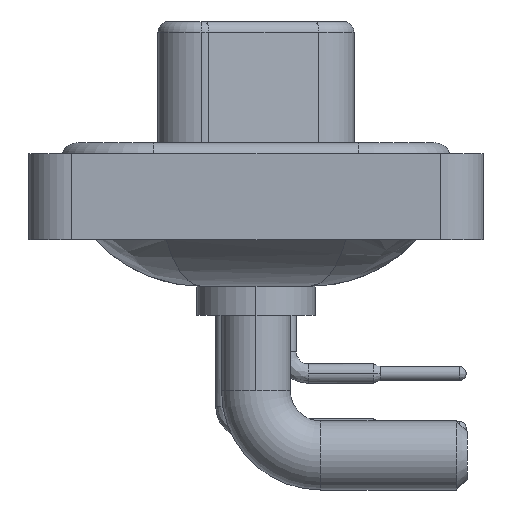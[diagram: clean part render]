
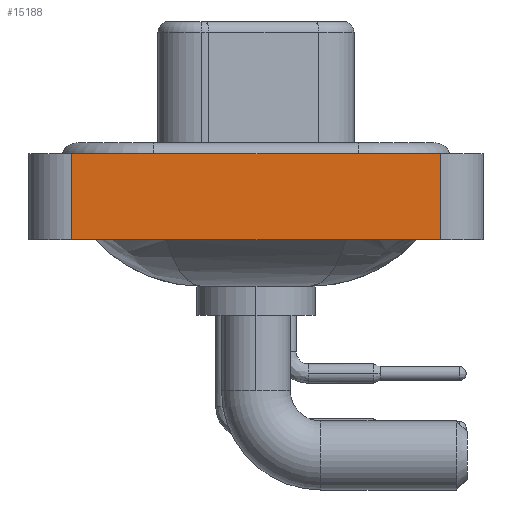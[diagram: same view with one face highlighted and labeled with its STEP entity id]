
A CAD part, left-side view. The second image highlights one B-rep face of the part: STEP entity #15188.
In plain terms, the highlighted planar face has unit normal (-1, 0, 0).
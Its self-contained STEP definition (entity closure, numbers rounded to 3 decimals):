
#983 = DIRECTION ( 'NONE',  ( -1., 0., 0. ) ) ;
#1183 = CARTESIAN_POINT ( 'NONE',  ( -7.35, -8.55, 0.4 ) ) ;
#1328 = EDGE_CURVE ( 'NONE', #18707, #13131, #21743, .T. ) ;
#1585 = EDGE_CURVE ( 'NONE', #18707, #22720, #2840, .T. ) ;
#2404 = EDGE_LOOP ( 'NONE', ( #7082, #12515, #13923, #10866 ) ) ;
#2840 = LINE ( 'NONE', #12979, #15301 ) ;
#2949 = FACE_OUTER_BOUND ( 'NONE', #2404, .T. ) ;
#3801 = VECTOR ( 'NONE', #6487, 1000. ) ;
#5107 = DIRECTION ( 'NONE',  ( 0., 0., 1. ) ) ;
#6487 = DIRECTION ( 'NONE',  ( 0., -1., 0. ) ) ;
#6903 = CARTESIAN_POINT ( 'NONE',  ( -7.35, -8.55, -3.6 ) ) ;
#7082 = ORIENTED_EDGE ( 'NONE', *, *, #14349, .T. ) ;
#7243 = CARTESIAN_POINT ( 'NONE',  ( -7.35, 8.55, -3.6 ) ) ;
#9019 = DIRECTION ( 'NONE',  ( 0., 0., 1. ) ) ;
#9281 = PLANE ( 'NONE',  #21381 ) ;
#10866 = ORIENTED_EDGE ( 'NONE', *, *, #1585, .T. ) ;
#11995 = EDGE_CURVE ( 'NONE', #13131, #23366, #19168, .T. ) ;
#12515 = ORIENTED_EDGE ( 'NONE', *, *, #11995, .F. ) ;
#12979 = CARTESIAN_POINT ( 'NONE',  ( -7.35, -8.55, -3.6 ) ) ;
#13131 = VERTEX_POINT ( 'NONE', #18249 ) ;
#13923 = ORIENTED_EDGE ( 'NONE', *, *, #1328, .F. ) ;
#14042 = VECTOR ( 'NONE', #5107, 1000. ) ;
#14349 = EDGE_CURVE ( 'NONE', #22720, #23366, #21097, .T. ) ;
#15188 = ADVANCED_FACE ( 'NONE', ( #2949 ), #9281, .T. ) ;
#15301 = VECTOR ( 'NONE', #22904, 1000. ) ;
#18144 = CARTESIAN_POINT ( 'NONE',  ( -7.35, 8.55, -3.6 ) ) ;
#18249 = CARTESIAN_POINT ( 'NONE',  ( -7.35, 8.55, 0.4 ) ) ;
#18707 = VERTEX_POINT ( 'NONE', #7243 ) ;
#19168 = LINE ( 'NONE', #25128, #3801 ) ;
#19378 = CARTESIAN_POINT ( 'NONE',  ( -7.35, -8.55, -3.6 ) ) ;
#19766 = DIRECTION ( 'NONE',  ( 0., 0., 1. ) ) ;
#19958 = CARTESIAN_POINT ( 'NONE',  ( -7.35, -8.55, -3.6 ) ) ;
#21097 = LINE ( 'NONE', #19378, #14042 ) ;
#21381 = AXIS2_PLACEMENT_3D ( 'NONE', #6903, #983, #9019 ) ;
#21743 = LINE ( 'NONE', #18144, #22311 ) ;
#22311 = VECTOR ( 'NONE', #19766, 1000. ) ;
#22720 = VERTEX_POINT ( 'NONE', #19958 ) ;
#22904 = DIRECTION ( 'NONE',  ( 0., -1., 0. ) ) ;
#23366 = VERTEX_POINT ( 'NONE', #1183 ) ;
#25128 = CARTESIAN_POINT ( 'NONE',  ( -7.35, -8.55, 0.4 ) ) ;
